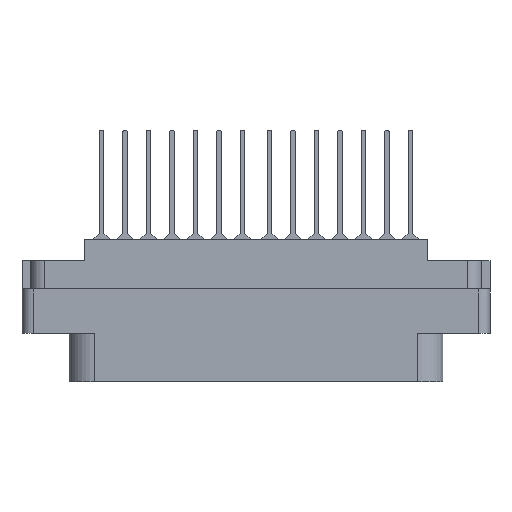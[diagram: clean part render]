
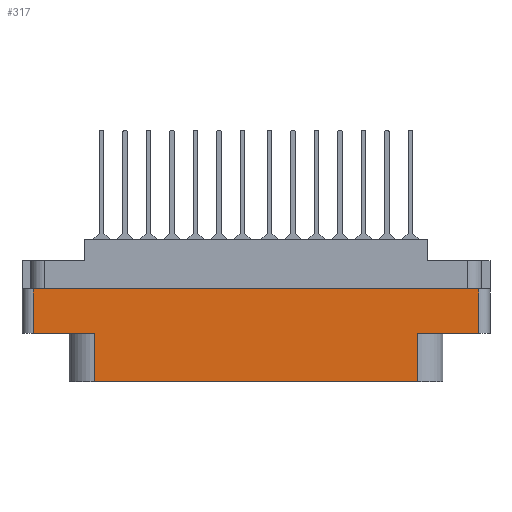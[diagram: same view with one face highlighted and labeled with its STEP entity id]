
A CAD part, front view. The second image highlights one B-rep face of the part: STEP entity #317.
In plain terms, the highlighted planar face has unit normal (0, -1, 0).
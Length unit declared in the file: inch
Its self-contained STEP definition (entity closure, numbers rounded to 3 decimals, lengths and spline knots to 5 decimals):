
#317 = ADVANCED_FACE ( 'NONE', ( #1211 ), #31784, .T. ) ;
#473 = LINE ( 'NONE', #7812, #24409 ) ;
#1047 = CARTESIAN_POINT ( 'NONE',  ( 0.895, -0.438, -0.52 ) ) ;
#1063 = ORIENTED_EDGE ( 'NONE', *, *, #12237, .T. ) ;
#1211 = FACE_OUTER_BOUND ( 'NONE', #35526, .T. ) ;
#2992 = CARTESIAN_POINT ( 'NONE',  ( -1.2335, -0.438, -0.52 ) ) ;
#3833 = ORIENTED_EDGE ( 'NONE', *, *, #24244, .T. ) ;
#4108 = LINE ( 'NONE', #30469, #46507 ) ;
#4364 = EDGE_CURVE ( 'NONE', #47344, #6309, #31759, .T. ) ;
#4667 = VERTEX_POINT ( 'NONE', #9656 ) ;
#5940 = EDGE_CURVE ( 'NONE', #28340, #7822, #4108, .T. ) ;
#5984 = CARTESIAN_POINT ( 'NONE',  ( -0.895, -0.438, -0.789 ) ) ;
#6309 = VERTEX_POINT ( 'NONE', #2992 ) ;
#6388 = EDGE_CURVE ( 'NONE', #28340, #6309, #473, .T. ) ;
#6554 = ORIENTED_EDGE ( 'NONE', *, *, #5940, .F. ) ;
#7812 = CARTESIAN_POINT ( 'NONE',  ( -1.2335, -0.438, -0.789 ) ) ;
#7822 = VERTEX_POINT ( 'NONE', #45232 ) ;
#9530 = VERTEX_POINT ( 'NONE', #5984 ) ;
#9656 = CARTESIAN_POINT ( 'NONE',  ( 0.895, -0.438, -0.789 ) ) ;
#11553 = VECTOR ( 'NONE', #14420, 39.37008 ) ;
#12017 = EDGE_CURVE ( 'NONE', #34675, #33415, #36667, .T. ) ;
#12022 = CARTESIAN_POINT ( 'NONE',  ( 1.2335, -0.438, -0.789 ) ) ;
#12164 = EDGE_CURVE ( 'NONE', #47344, #9530, #18733, .T. ) ;
#12237 = EDGE_CURVE ( 'NONE', #9530, #4667, #19921, .T. ) ;
#12635 = CARTESIAN_POINT ( 'NONE',  ( 1.2335, -0.438, -0.52 ) ) ;
#13607 = CARTESIAN_POINT ( 'NONE',  ( 0.895, -0.438, -0.52 ) ) ;
#14420 = DIRECTION ( 'NONE',  ( -1., 0., 0. ) ) ;
#15104 = DIRECTION ( 'NONE',  ( 1., 0., 0. ) ) ;
#15680 = CARTESIAN_POINT ( 'NONE',  ( -1.2335, -0.438, -0.274 ) ) ;
#15755 = DIRECTION ( 'NONE',  ( 0., 0., -1. ) ) ;
#15899 = CARTESIAN_POINT ( 'NONE',  ( -0.895, -0.438, -0.52 ) ) ;
#16190 = DIRECTION ( 'NONE',  ( 0., 0., -1. ) ) ;
#16853 = VECTOR ( 'NONE', #40826, 39.37008 ) ;
#18064 = VECTOR ( 'NONE', #46592, 39.37008 ) ;
#18278 = CARTESIAN_POINT ( 'NONE',  ( 0., -0.438, -0.52 ) ) ;
#18733 = LINE ( 'NONE', #33982, #34268 ) ;
#19921 = LINE ( 'NONE', #27394, #33019 ) ;
#19986 = VECTOR ( 'NONE', #31487, 39.37008 ) ;
#21036 = AXIS2_PLACEMENT_3D ( 'NONE', #34849, #38667, #15755 ) ;
#24244 = EDGE_CURVE ( 'NONE', #4667, #33415, #31340, .T. ) ;
#24409 = VECTOR ( 'NONE', #16190, 39.37008 ) ;
#25865 = ORIENTED_EDGE ( 'NONE', *, *, #12164, .T. ) ;
#27394 = CARTESIAN_POINT ( 'NONE',  ( -1.2955, -0.438, -0.789 ) ) ;
#28340 = VERTEX_POINT ( 'NONE', #15680 ) ;
#30469 = CARTESIAN_POINT ( 'NONE',  ( 0., -0.438, -0.274 ) ) ;
#31340 = LINE ( 'NONE', #1047, #19986 ) ;
#31487 = DIRECTION ( 'NONE',  ( 0., 0., 1. ) ) ;
#31759 = LINE ( 'NONE', #40170, #16853 ) ;
#31761 = DIRECTION ( 'NONE',  ( 1., 0., 0. ) ) ;
#31784 = PLANE ( 'NONE',  #21036 ) ;
#32704 = ORIENTED_EDGE ( 'NONE', *, *, #44882, .T. ) ;
#33019 = VECTOR ( 'NONE', #31761, 39.37008 ) ;
#33415 = VERTEX_POINT ( 'NONE', #13607 ) ;
#33810 = ORIENTED_EDGE ( 'NONE', *, *, #6388, .T. ) ;
#33982 = CARTESIAN_POINT ( 'NONE',  ( -0.895, -0.438, -0.789 ) ) ;
#34268 = VECTOR ( 'NONE', #37835, 39.37008 ) ;
#34675 = VERTEX_POINT ( 'NONE', #12635 ) ;
#34837 = LINE ( 'NONE', #12022, #18064 ) ;
#34849 = CARTESIAN_POINT ( 'NONE',  ( -1.2955, -0.438, -0.789 ) ) ;
#35472 = ORIENTED_EDGE ( 'NONE', *, *, #12017, .F. ) ;
#35526 = EDGE_LOOP ( 'NONE', ( #6554, #33810, #37526, #25865, #1063, #3833, #35472, #32704 ) ) ;
#36667 = LINE ( 'NONE', #18278, #11553 ) ;
#37526 = ORIENTED_EDGE ( 'NONE', *, *, #4364, .F. ) ;
#37835 = DIRECTION ( 'NONE',  ( 0., 0., -1. ) ) ;
#38667 = DIRECTION ( 'NONE',  ( 0., -1., 0. ) ) ;
#40170 = CARTESIAN_POINT ( 'NONE',  ( 0., -0.438, -0.52 ) ) ;
#40826 = DIRECTION ( 'NONE',  ( -1., 0., 0. ) ) ;
#44882 = EDGE_CURVE ( 'NONE', #34675, #7822, #34837, .T. ) ;
#45232 = CARTESIAN_POINT ( 'NONE',  ( 1.2335, -0.438, -0.274 ) ) ;
#46507 = VECTOR ( 'NONE', #15104, 39.37008 ) ;
#46592 = DIRECTION ( 'NONE',  ( 0., 0., 1. ) ) ;
#47344 = VERTEX_POINT ( 'NONE', #15899 ) ;
